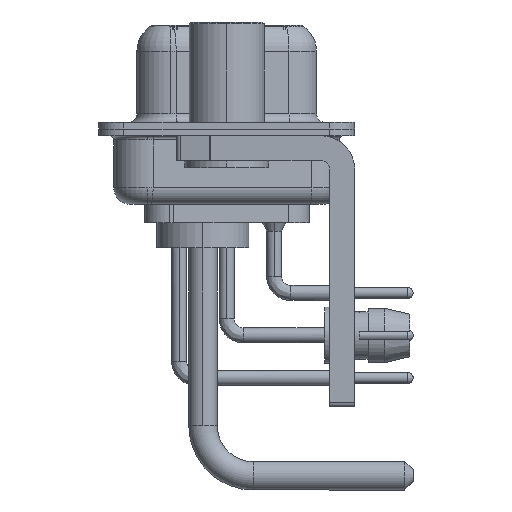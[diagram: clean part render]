
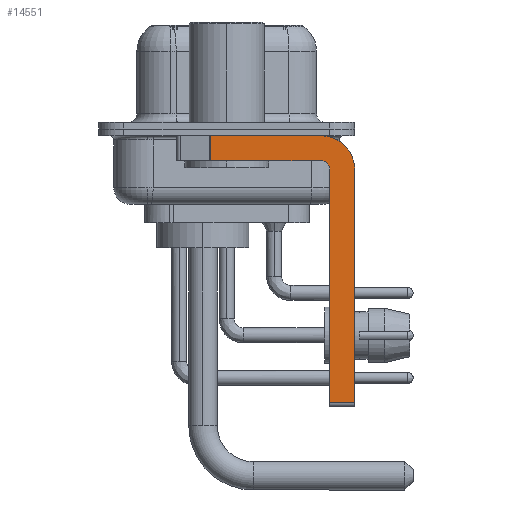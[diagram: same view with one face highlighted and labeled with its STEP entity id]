
A CAD part, left-side view. The second image highlights one B-rep face of the part: STEP entity #14551.
In plain terms, the highlighted planar face has unit normal (-1, 0, 0).
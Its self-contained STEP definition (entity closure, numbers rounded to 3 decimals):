
#84 = EDGE_CURVE ( 'NONE', #25126, #27499, #19443, .T. ) ;
#346 = ORIENTED_EDGE ( 'NONE', *, *, #23427, .F. ) ;
#404 = CARTESIAN_POINT ( 'NONE',  ( -2.9, 0.978, -0.4 ) ) ;
#2249 = CIRCLE ( 'NONE', #13618, 0.5 ) ;
#2554 = CARTESIAN_POINT ( 'NONE',  ( -2.9, -5.65, -1.9 ) ) ;
#3306 = DIRECTION ( 'NONE',  ( 0., 0., -1. ) ) ;
#3936 = DIRECTION ( 'NONE',  ( 1., 0., 0. ) ) ;
#5599 = VERTEX_POINT ( 'NONE', #28413 ) ;
#5677 = LINE ( 'NONE', #13300, #17411 ) ;
#5761 = DIRECTION ( 'NONE',  ( -1., 0., 0. ) ) ;
#6185 = CARTESIAN_POINT ( 'NONE',  ( -2.9, -5.65, -2.4 ) ) ;
#6825 = VERTEX_POINT ( 'NONE', #10289 ) ;
#8823 = LINE ( 'NONE', #21344, #26320 ) ;
#9170 = CARTESIAN_POINT ( 'NONE',  ( -2.9, -5.65, -0.4 ) ) ;
#10002 = ORIENTED_EDGE ( 'NONE', *, *, #10966, .F. ) ;
#10289 = CARTESIAN_POINT ( 'NONE',  ( -2.9, -7.65, -2.4 ) ) ;
#10665 = CARTESIAN_POINT ( 'NONE',  ( -2.9, -5.65, -2.4 ) ) ;
#10966 = EDGE_CURVE ( 'NONE', #29493, #6825, #25515, .T. ) ;
#11898 = DIRECTION ( 'NONE',  ( 0., 0., -1. ) ) ;
#12160 = EDGE_CURVE ( 'NONE', #33154, #5599, #19193, .T. ) ;
#13207 = DIRECTION ( 'NONE',  ( 0., 0., 1. ) ) ;
#13300 = CARTESIAN_POINT ( 'NONE',  ( -2.9, -7.65, -2.4 ) ) ;
#13618 = AXIS2_PLACEMENT_3D ( 'NONE', #10665, #5761, #13207 ) ;
#14184 = DIRECTION ( 'NONE',  ( 0., 0., -1. ) ) ;
#14551 = ADVANCED_FACE ( 'NONE', ( #18898 ), #29237, .F. ) ;
#14686 = CARTESIAN_POINT ( 'NONE',  ( -2.9, 0.978, -1.9 ) ) ;
#14762 = VERTEX_POINT ( 'NONE', #32597 ) ;
#15309 = VECTOR ( 'NONE', #24448, 1000. ) ;
#15757 = ORIENTED_EDGE ( 'NONE', *, *, #19912, .F. ) ;
#16172 = DIRECTION ( 'NONE',  ( 0., 0., -1. ) ) ;
#16792 = EDGE_CURVE ( 'NONE', #27712, #27499, #8823, .T. ) ;
#17411 = VECTOR ( 'NONE', #3306, 1000. ) ;
#18898 = FACE_OUTER_BOUND ( 'NONE', #28546, .T. ) ;
#18931 = LINE ( 'NONE', #27222, #30475 ) ;
#19193 = LINE ( 'NONE', #26473, #15309 ) ;
#19443 = LINE ( 'NONE', #14686, #33443 ) ;
#19643 = ORIENTED_EDGE ( 'NONE', *, *, #24772, .T. ) ;
#19912 = EDGE_CURVE ( 'NONE', #25126, #29493, #24559, .T. ) ;
#21344 = CARTESIAN_POINT ( 'NONE',  ( -2.9, -5.65, -1.9 ) ) ;
#21609 = EDGE_CURVE ( 'NONE', #5599, #27712, #2249, .T. ) ;
#21786 = DIRECTION ( 'NONE',  ( 0., -1., 0. ) ) ;
#21990 = CARTESIAN_POINT ( 'NONE',  ( -2.9, 3., -0.4 ) ) ;
#22165 = ORIENTED_EDGE ( 'NONE', *, *, #84, .T. ) ;
#22687 = ORIENTED_EDGE ( 'NONE', *, *, #16792, .F. ) ;
#23427 = EDGE_CURVE ( 'NONE', #6825, #14762, #5677, .T. ) ;
#23900 = DIRECTION ( 'NONE',  ( 0., 1., 0. ) ) ;
#24448 = DIRECTION ( 'NONE',  ( 0., 0., 1. ) ) ;
#24559 = LINE ( 'NONE', #21990, #31368 ) ;
#24772 = EDGE_CURVE ( 'NONE', #33154, #14762, #18931, .T. ) ;
#25126 = VERTEX_POINT ( 'NONE', #404 ) ;
#25515 = CIRCLE ( 'NONE', #27162, 2. ) ;
#26011 = CARTESIAN_POINT ( 'NONE',  ( -2.9, 0.978, -1.9 ) ) ;
#26320 = VECTOR ( 'NONE', #23900, 1000. ) ;
#26473 = CARTESIAN_POINT ( 'NONE',  ( -2.9, -6.15, -16.6 ) ) ;
#26681 = DIRECTION ( 'NONE',  ( 1., 0., 0. ) ) ;
#27162 = AXIS2_PLACEMENT_3D ( 'NONE', #29866, #3936, #11898 ) ;
#27222 = CARTESIAN_POINT ( 'NONE',  ( -2.9, -5.65, -16.35 ) ) ;
#27499 = VERTEX_POINT ( 'NONE', #26011 ) ;
#27712 = VERTEX_POINT ( 'NONE', #2554 ) ;
#28413 = CARTESIAN_POINT ( 'NONE',  ( -2.9, -6.15, -2.4 ) ) ;
#28546 = EDGE_LOOP ( 'NONE', ( #15757, #22165, #22687, #29950, #33390, #19643, #346, #10002 ) ) ;
#29237 = PLANE ( 'NONE',  #29961 ) ;
#29493 = VERTEX_POINT ( 'NONE', #9170 ) ;
#29866 = CARTESIAN_POINT ( 'NONE',  ( -2.9, -5.65, -2.4 ) ) ;
#29950 = ORIENTED_EDGE ( 'NONE', *, *, #21609, .F. ) ;
#29961 = AXIS2_PLACEMENT_3D ( 'NONE', #6185, #26681, #16172 ) ;
#30475 = VECTOR ( 'NONE', #21786, 1000. ) ;
#31368 = VECTOR ( 'NONE', #32157, 1000. ) ;
#31481 = CARTESIAN_POINT ( 'NONE',  ( -2.9, -6.15, -16.35 ) ) ;
#32157 = DIRECTION ( 'NONE',  ( 0., -1., 0. ) ) ;
#32597 = CARTESIAN_POINT ( 'NONE',  ( -2.9, -7.65, -16.35 ) ) ;
#33154 = VERTEX_POINT ( 'NONE', #31481 ) ;
#33390 = ORIENTED_EDGE ( 'NONE', *, *, #12160, .F. ) ;
#33443 = VECTOR ( 'NONE', #14184, 1000. ) ;
